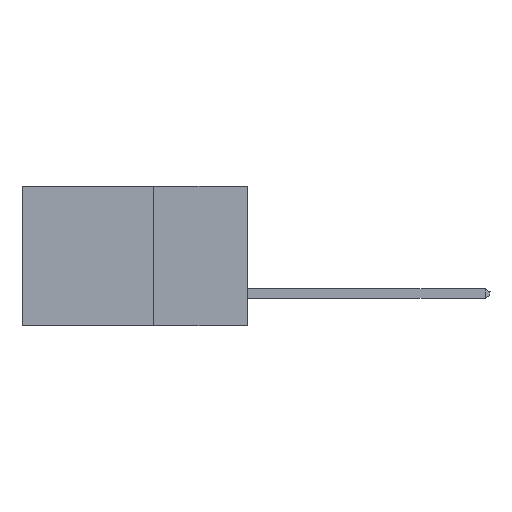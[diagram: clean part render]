
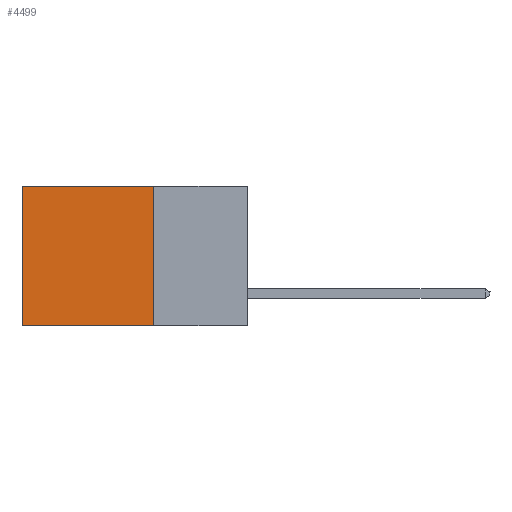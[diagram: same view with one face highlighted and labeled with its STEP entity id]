
A CAD part, left-side view. The second image highlights one B-rep face of the part: STEP entity #4499.
In plain terms, the highlighted planar face has unit normal (-1, 0, 0).
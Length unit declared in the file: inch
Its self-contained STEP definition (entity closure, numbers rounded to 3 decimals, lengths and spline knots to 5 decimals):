
#193 = VECTOR ( 'NONE', #7675, 39.37008 ) ;
#516 = CARTESIAN_POINT ( 'NONE',  ( 0.2615, 0.25, -0.37 ) ) ;
#752 = DIRECTION ( 'NONE',  ( 0., 1., 0. ) ) ;
#894 = DIRECTION ( 'NONE',  ( 0., 0., -1. ) ) ;
#904 = DIRECTION ( 'NONE',  ( 0., 0., -1. ) ) ;
#1032 = DIRECTION ( 'NONE',  ( 1., 0., 0. ) ) ;
#1292 = AXIS2_PLACEMENT_3D ( 'NONE', #12247, #1032, #894 ) ;
#1753 = VERTEX_POINT ( 'NONE', #8858 ) ;
#1894 = CARTESIAN_POINT ( 'NONE',  ( 0.2615, 0.25, -0.37 ) ) ;
#1904 = CARTESIAN_POINT ( 'NONE',  ( 0.2615, 0.6, -0.37 ) ) ;
#2045 = VERTEX_POINT ( 'NONE', #516 ) ;
#2250 = EDGE_CURVE ( 'NONE', #4694, #1753, #9108, .T. ) ;
#2772 = LINE ( 'NONE', #4897, #5909 ) ;
#3390 = VECTOR ( 'NONE', #752, 39.37008 ) ;
#3631 = CARTESIAN_POINT ( 'NONE',  ( 0.2615, 0.6, -0.37 ) ) ;
#4215 = EDGE_CURVE ( 'NONE', #4694, #2045, #2772, .T. ) ;
#4499 = ADVANCED_FACE ( 'NONE', ( #13161 ), #8077, .F. ) ;
#4694 = VERTEX_POINT ( 'NONE', #8730 ) ;
#4897 = CARTESIAN_POINT ( 'NONE',  ( 0.2615, 0.25, -0.37 ) ) ;
#5687 = ORIENTED_EDGE ( 'NONE', *, *, #11865, .T. ) ;
#5909 = VECTOR ( 'NONE', #904, 39.37008 ) ;
#7675 = DIRECTION ( 'NONE',  ( 0., 0., -1. ) ) ;
#8057 = ORIENTED_EDGE ( 'NONE', *, *, #4215, .F. ) ;
#8077 = PLANE ( 'NONE',  #1292 ) ;
#8730 = CARTESIAN_POINT ( 'NONE',  ( 0.2615, 0.25, 0. ) ) ;
#8858 = CARTESIAN_POINT ( 'NONE',  ( 0.2615, 0.6, 0. ) ) ;
#8872 = LINE ( 'NONE', #1894, #3390 ) ;
#8892 = ORIENTED_EDGE ( 'NONE', *, *, #9673, .F. ) ;
#9108 = LINE ( 'NONE', #12354, #9640 ) ;
#9640 = VECTOR ( 'NONE', #11255, 39.37008 ) ;
#9673 = EDGE_CURVE ( 'NONE', #2045, #10371, #8872, .T. ) ;
#10371 = VERTEX_POINT ( 'NONE', #1904 ) ;
#11178 = EDGE_LOOP ( 'NONE', ( #5687, #8892, #8057, #12671 ) ) ;
#11255 = DIRECTION ( 'NONE',  ( 0., 1., 0. ) ) ;
#11865 = EDGE_CURVE ( 'NONE', #1753, #10371, #12696, .T. ) ;
#12247 = CARTESIAN_POINT ( 'NONE',  ( 0.2615, 0.25, -0.37 ) ) ;
#12354 = CARTESIAN_POINT ( 'NONE',  ( 0.2615, 0.25, 0. ) ) ;
#12671 = ORIENTED_EDGE ( 'NONE', *, *, #2250, .T. ) ;
#12696 = LINE ( 'NONE', #3631, #193 ) ;
#13161 = FACE_OUTER_BOUND ( 'NONE', #11178, .T. ) ;
